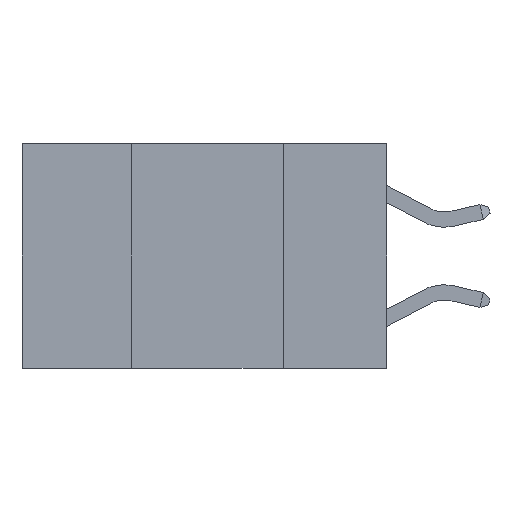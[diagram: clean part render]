
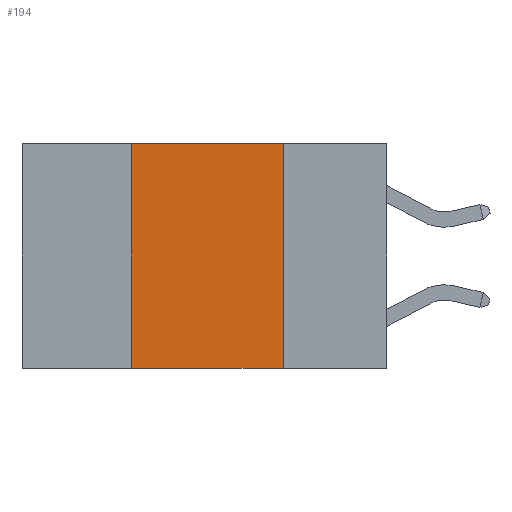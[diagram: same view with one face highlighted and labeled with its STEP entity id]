
A CAD part, left-side view. The second image highlights one B-rep face of the part: STEP entity #194.
In plain terms, the highlighted planar face has unit normal (-1, 0, 0).
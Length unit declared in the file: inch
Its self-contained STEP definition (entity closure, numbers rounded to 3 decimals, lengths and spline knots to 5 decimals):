
#194 = ADVANCED_FACE ( 'NONE', ( #5969 ), #4619, .F. ) ;
#550 = LINE ( 'NONE', #4247, #7213 ) ;
#755 = EDGE_CURVE ( 'NONE', #10772, #1605, #8677, .T. ) ;
#769 = EDGE_CURVE ( 'NONE', #1251, #968, #3819, .T. ) ;
#968 = VERTEX_POINT ( 'NONE', #3596 ) ;
#1251 = VERTEX_POINT ( 'NONE', #6177 ) ;
#1479 = CARTESIAN_POINT ( 'NONE',  ( 0., 0.6, 0. ) ) ;
#1605 = VERTEX_POINT ( 'NONE', #6125 ) ;
#2732 = DIRECTION ( 'NONE',  ( 0., -1., 0. ) ) ;
#3331 = CARTESIAN_POINT ( 'NONE',  ( 0., 0.6, 0. ) ) ;
#3440 = DIRECTION ( 'NONE',  ( 0., 0., -1. ) ) ;
#3596 = CARTESIAN_POINT ( 'NONE',  ( 0., 0.17, -0.37 ) ) ;
#3819 = LINE ( 'NONE', #8981, #10790 ) ;
#4175 = ORIENTED_EDGE ( 'NONE', *, *, #10080, .F. ) ;
#4247 = CARTESIAN_POINT ( 'NONE',  ( 0., 0.17, 0. ) ) ;
#4619 = PLANE ( 'NONE',  #9635 ) ;
#4771 = LINE ( 'NONE', #4933, #9333 ) ;
#4931 = DIRECTION ( 'NONE',  ( 1., 0., 0. ) ) ;
#4933 = CARTESIAN_POINT ( 'NONE',  ( 0., 0.42, 0. ) ) ;
#5969 = FACE_OUTER_BOUND ( 'NONE', #11234, .T. ) ;
#6103 = DIRECTION ( 'NONE',  ( 0., 0., -1. ) ) ;
#6125 = CARTESIAN_POINT ( 'NONE',  ( 0., 0.17, 0. ) ) ;
#6177 = CARTESIAN_POINT ( 'NONE',  ( 0., 0.42, -0.37 ) ) ;
#6236 = VECTOR ( 'NONE', #2732, 39.37008 ) ;
#7213 = VECTOR ( 'NONE', #6103, 39.37008 ) ;
#7946 = CARTESIAN_POINT ( 'NONE',  ( 0., 0.42, 0. ) ) ;
#8572 = DIRECTION ( 'NONE',  ( 0., 0., 1. ) ) ;
#8677 = LINE ( 'NONE', #1479, #6236 ) ;
#8898 = DIRECTION ( 'NONE',  ( 0., -1., 0. ) ) ;
#8981 = CARTESIAN_POINT ( 'NONE',  ( 0., 0.6, -0.37 ) ) ;
#9333 = VECTOR ( 'NONE', #8572, 39.37008 ) ;
#9340 = ORIENTED_EDGE ( 'NONE', *, *, #755, .F. ) ;
#9592 = ORIENTED_EDGE ( 'NONE', *, *, #769, .T. ) ;
#9635 = AXIS2_PLACEMENT_3D ( 'NONE', #3331, #4931, #3440 ) ;
#10080 = EDGE_CURVE ( 'NONE', #1605, #968, #550, .T. ) ;
#10592 = EDGE_CURVE ( 'NONE', #1251, #10772, #4771, .T. ) ;
#10772 = VERTEX_POINT ( 'NONE', #7946 ) ;
#10790 = VECTOR ( 'NONE', #8898, 39.37008 ) ;
#11234 = EDGE_LOOP ( 'NONE', ( #4175, #9340, #11392, #9592 ) ) ;
#11392 = ORIENTED_EDGE ( 'NONE', *, *, #10592, .F. ) ;
